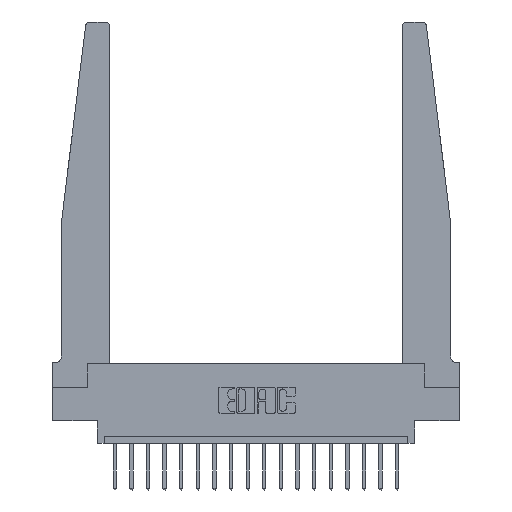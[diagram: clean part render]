
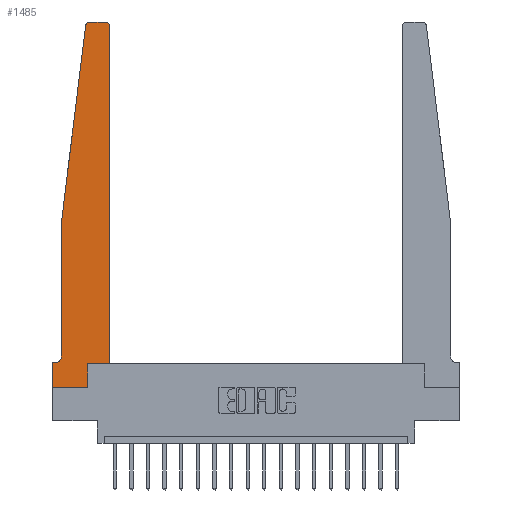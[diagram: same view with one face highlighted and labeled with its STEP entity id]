
A CAD part, top view. The second image highlights one B-rep face of the part: STEP entity #1485.
In plain terms, the highlighted planar face has unit normal (0, 0, 1).
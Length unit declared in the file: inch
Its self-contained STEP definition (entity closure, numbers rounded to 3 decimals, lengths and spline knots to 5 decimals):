
#13 = CARTESIAN_POINT ( 'NONE',  ( 0., 0., 0.37 ) ) ;
#229 = ORIENTED_EDGE ( 'NONE', *, *, #11741, .T. ) ;
#335 = CARTESIAN_POINT ( 'NONE',  ( 0.015, 0.1875, 0.37 ) ) ;
#410 = DIRECTION ( 'NONE',  ( -1., 0., 0. ) ) ;
#632 = EDGE_CURVE ( 'NONE', #8645, #10507, #9144, .T. ) ;
#1082 = DIRECTION ( 'NONE',  ( 0., 0., 1. ) ) ;
#1306 = CARTESIAN_POINT ( 'NONE',  ( 0., 0.1875, 0.37 ) ) ;
#1485 = ADVANCED_FACE ( 'NONE', ( #9585 ), #11908, .T. ) ;
#1538 = VERTEX_POINT ( 'NONE', #7809 ) ;
#1593 = DIRECTION ( 'NONE',  ( 0., -1., 0. ) ) ;
#2071 = CARTESIAN_POINT ( 'NONE',  ( 0.395, 2.72, 0.37 ) ) ;
#2098 = LINE ( 'NONE', #7902, #7689 ) ;
#2322 = VERTEX_POINT ( 'NONE', #7879 ) ;
#2370 = VECTOR ( 'NONE', #16834, 39.37008 ) ;
#2404 = CARTESIAN_POINT ( 'NONE',  ( 0.395, 2.75, 0.37 ) ) ;
#2782 = ORIENTED_EDGE ( 'NONE', *, *, #14326, .T. ) ;
#2951 = DIRECTION ( 'NONE',  ( 0., 0., 1. ) ) ;
#2999 = LINE ( 'NONE', #5733, #6473 ) ;
#3223 = LINE ( 'NONE', #14284, #17227 ) ;
#3240 = ORIENTED_EDGE ( 'NONE', *, *, #632, .T. ) ;
#3252 = EDGE_CURVE ( 'NONE', #18337, #8645, #7141, .T. ) ;
#3253 = CARTESIAN_POINT ( 'NONE',  ( 0.425, 0.18, 0.37 ) ) ;
#3282 = VECTOR ( 'NONE', #1593, 39.37008 ) ;
#3345 = CARTESIAN_POINT ( 'NONE',  ( 0., 0., 0.37 ) ) ;
#3629 = LINE ( 'NONE', #16033, #4984 ) ;
#3763 = DIRECTION ( 'NONE',  ( 1., 0., 0. ) ) ;
#4685 = CARTESIAN_POINT ( 'NONE',  ( 0.425, 2.72, 0.37 ) ) ;
#4819 = ORIENTED_EDGE ( 'NONE', *, *, #16893, .T. ) ;
#4984 = VECTOR ( 'NONE', #14606, 39.37008 ) ;
#5015 = EDGE_CURVE ( 'NONE', #7282, #16873, #5726, .T. ) ;
#5031 = CARTESIAN_POINT ( 'NONE',  ( 0.065, 0.1875, 0.37 ) ) ;
#5035 = DIRECTION ( 'NONE',  ( 1., 0., 0. ) ) ;
#5123 = CARTESIAN_POINT ( 'NONE',  ( 0.425, 0.18, 0.37 ) ) ;
#5587 = LINE ( 'NONE', #13673, #3282 ) ;
#5726 = CIRCLE ( 'NONE', #18441, 0.03 ) ;
#5733 = CARTESIAN_POINT ( 'NONE',  ( 0.065, 1.25, 0.37 ) ) ;
#6044 = ORIENTED_EDGE ( 'NONE', *, *, #15472, .T. ) ;
#6134 = ORIENTED_EDGE ( 'NONE', *, *, #13530, .T. ) ;
#6262 = CARTESIAN_POINT ( 'NONE',  ( 0.2605, 0.18, 0.37 ) ) ;
#6473 = VECTOR ( 'NONE', #13080, 39.37008 ) ;
#7001 = DIRECTION ( 'NONE',  ( 1., 0., 0. ) ) ;
#7132 = VERTEX_POINT ( 'NONE', #13829 ) ;
#7141 = CIRCLE ( 'NONE', #10296, 0.05 ) ;
#7282 = VERTEX_POINT ( 'NONE', #4685 ) ;
#7299 = AXIS2_PLACEMENT_3D ( 'NONE', #14201, #1082, #7001 ) ;
#7689 = VECTOR ( 'NONE', #10812, 39.37008 ) ;
#7809 = CARTESIAN_POINT ( 'NONE',  ( 0.2605, 0.18, 0.37 ) ) ;
#7879 = CARTESIAN_POINT ( 'NONE',  ( 0.27653, 2.75, 0.37 ) ) ;
#7902 = CARTESIAN_POINT ( 'NONE',  ( 0.25, 2.75, 0.37 ) ) ;
#8108 = VECTOR ( 'NONE', #17901, 39.37008 ) ;
#8165 = VERTEX_POINT ( 'NONE', #3253 ) ;
#8367 = EDGE_LOOP ( 'NONE', ( #6134, #6044, #16195, #8588, #15845, #3240, #4819, #9939, #2782, #18040, #229, #11570 ) ) ;
#8588 = ORIENTED_EDGE ( 'NONE', *, *, #8983, .T. ) ;
#8645 = VERTEX_POINT ( 'NONE', #335 ) ;
#8983 = EDGE_CURVE ( 'NONE', #14029, #18337, #5587, .T. ) ;
#9144 = LINE ( 'NONE', #5031, #2370 ) ;
#9183 = VERTEX_POINT ( 'NONE', #3345 ) ;
#9440 = CARTESIAN_POINT ( 'NONE',  ( 0.065, 1.25, 0.37 ) ) ;
#9585 = FACE_OUTER_BOUND ( 'NONE', #8367, .T. ) ;
#9670 = VECTOR ( 'NONE', #15596, 39.37008 ) ;
#9939 = ORIENTED_EDGE ( 'NONE', *, *, #14802, .T. ) ;
#10051 = EDGE_CURVE ( 'NONE', #15699, #14029, #2999, .T. ) ;
#10163 = CARTESIAN_POINT ( 'NONE',  ( 0.24675, 2.72367, 0.37 ) ) ;
#10270 = DIRECTION ( 'NONE',  ( 1., 0., 0. ) ) ;
#10296 = AXIS2_PLACEMENT_3D ( 'NONE', #12459, #15408, #410 ) ;
#10507 = VERTEX_POINT ( 'NONE', #14021 ) ;
#10812 = DIRECTION ( 'NONE',  ( -1., 0., 0. ) ) ;
#11570 = ORIENTED_EDGE ( 'NONE', *, *, #5015, .T. ) ;
#11741 = EDGE_CURVE ( 'NONE', #8165, #7282, #15239, .T. ) ;
#11908 = PLANE ( 'NONE',  #14768 ) ;
#12119 = CIRCLE ( 'NONE', #7299, 0.03 ) ;
#12459 = CARTESIAN_POINT ( 'NONE',  ( 0.015, 0.2375, 0.37 ) ) ;
#12548 = DIRECTION ( 'NONE',  ( 0., 0., 1. ) ) ;
#12856 = LINE ( 'NONE', #6262, #8108 ) ;
#13080 = DIRECTION ( 'NONE',  ( -0.122, -0.992, 0. ) ) ;
#13530 = EDGE_CURVE ( 'NONE', #16873, #2322, #2098, .T. ) ;
#13673 = CARTESIAN_POINT ( 'NONE',  ( 0.065, 1.25, 0.37 ) ) ;
#13829 = CARTESIAN_POINT ( 'NONE',  ( 0.2605, 0., 0.37 ) ) ;
#14021 = CARTESIAN_POINT ( 'NONE',  ( 0., 0.1875, 0.37 ) ) ;
#14029 = VERTEX_POINT ( 'NONE', #9440 ) ;
#14201 = CARTESIAN_POINT ( 'NONE',  ( 0.27653, 2.72, 0.37 ) ) ;
#14215 = VECTOR ( 'NONE', #14955, 39.37008 ) ;
#14284 = CARTESIAN_POINT ( 'NONE',  ( 0.425, 0.18, 0.37 ) ) ;
#14326 = EDGE_CURVE ( 'NONE', #7132, #1538, #12856, .T. ) ;
#14606 = DIRECTION ( 'NONE',  ( 0., -1., 0. ) ) ;
#14768 = AXIS2_PLACEMENT_3D ( 'NONE', #1306, #2951, #10270 ) ;
#14802 = EDGE_CURVE ( 'NONE', #9183, #7132, #18877, .T. ) ;
#14955 = DIRECTION ( 'NONE',  ( 1., 0., 0. ) ) ;
#15239 = LINE ( 'NONE', #5123, #9670 ) ;
#15408 = DIRECTION ( 'NONE',  ( 0., 0., -1. ) ) ;
#15472 = EDGE_CURVE ( 'NONE', #2322, #15699, #12119, .T. ) ;
#15477 = CARTESIAN_POINT ( 'NONE',  ( 0.065, 0.2375, 0.37 ) ) ;
#15596 = DIRECTION ( 'NONE',  ( 0., 1., 0. ) ) ;
#15699 = VERTEX_POINT ( 'NONE', #10163 ) ;
#15845 = ORIENTED_EDGE ( 'NONE', *, *, #3252, .T. ) ;
#16033 = CARTESIAN_POINT ( 'NONE',  ( 0., 0., 0.37 ) ) ;
#16195 = ORIENTED_EDGE ( 'NONE', *, *, #10051, .T. ) ;
#16834 = DIRECTION ( 'NONE',  ( -1., 0., 0. ) ) ;
#16873 = VERTEX_POINT ( 'NONE', #2404 ) ;
#16893 = EDGE_CURVE ( 'NONE', #10507, #9183, #3629, .T. ) ;
#17227 = VECTOR ( 'NONE', #3763, 39.37008 ) ;
#17901 = DIRECTION ( 'NONE',  ( 0., 1., 0. ) ) ;
#18040 = ORIENTED_EDGE ( 'NONE', *, *, #18950, .T. ) ;
#18337 = VERTEX_POINT ( 'NONE', #15477 ) ;
#18441 = AXIS2_PLACEMENT_3D ( 'NONE', #2071, #12548, #5035 ) ;
#18877 = LINE ( 'NONE', #13, #14215 ) ;
#18950 = EDGE_CURVE ( 'NONE', #1538, #8165, #3223, .T. ) ;
